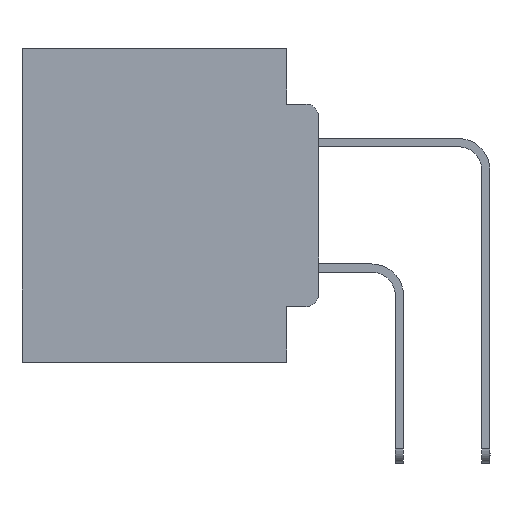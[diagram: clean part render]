
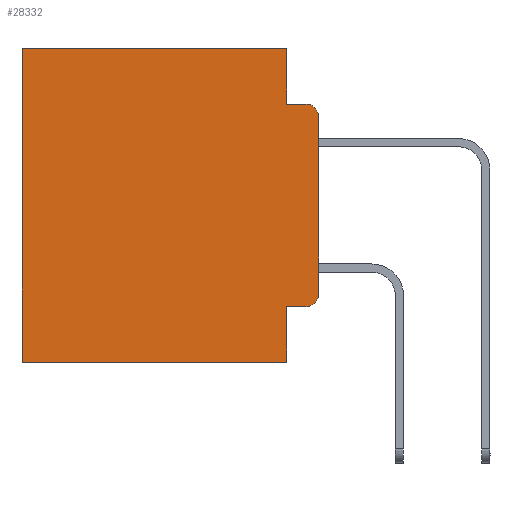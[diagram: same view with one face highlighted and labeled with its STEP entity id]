
A CAD part, left-side view. The second image highlights one B-rep face of the part: STEP entity #28332.
In plain terms, the highlighted planar face has unit normal (-1, 0, 0).
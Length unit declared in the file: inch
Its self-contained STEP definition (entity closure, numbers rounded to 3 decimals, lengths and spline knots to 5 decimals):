
#144 = LINE ( 'NONE', #2661, #5308 ) ;
#351 = VECTOR ( 'NONE', #19358, 39.37008 ) ;
#422 = LINE ( 'NONE', #11580, #24230 ) ;
#603 = EDGE_CURVE ( 'NONE', #9989, #10179, #6033, .T. ) ;
#659 = VERTEX_POINT ( 'NONE', #17639 ) ;
#731 = CARTESIAN_POINT ( 'NONE',  ( 0.298, 0.02, -0.3915 ) ) ;
#874 = VERTEX_POINT ( 'NONE', #2726 ) ;
#1506 = ORIENTED_EDGE ( 'NONE', *, *, #21153, .F. ) ;
#1819 = EDGE_LOOP ( 'NONE', ( #4537, #8935, #4600, #10059, #7791, #8073, #1506, #4955, #15226, #27487 ) ) ;
#2366 = DIRECTION ( 'NONE',  ( 0., 0., -1. ) ) ;
#2438 = DIRECTION ( 'NONE',  ( -1., 0., 0. ) ) ;
#2661 = CARTESIAN_POINT ( 'NONE',  ( 0.298, 0.051, 0. ) ) ;
#2663 = CARTESIAN_POINT ( 'NONE',  ( 0.298, 0., -0.1085 ) ) ;
#2726 = CARTESIAN_POINT ( 'NONE',  ( 0.298, 0.02, -0.4115 ) ) ;
#3197 = EDGE_CURVE ( 'NONE', #4149, #874, #23065, .T. ) ;
#3480 = CARTESIAN_POINT ( 'NONE',  ( 0.298, 0.473, 0. ) ) ;
#3643 = CARTESIAN_POINT ( 'NONE',  ( 0.298, 0.051, 0. ) ) ;
#4064 = VERTEX_POINT ( 'NONE', #20189 ) ;
#4145 = CARTESIAN_POINT ( 'NONE',  ( 0.298, 0., 0. ) ) ;
#4149 = VERTEX_POINT ( 'NONE', #6026 ) ;
#4158 = AXIS2_PLACEMENT_3D ( 'NONE', #731, #27908, #25831 ) ;
#4445 = CARTESIAN_POINT ( 'NONE',  ( 0.298, 0.473, 0. ) ) ;
#4537 = ORIENTED_EDGE ( 'NONE', *, *, #15327, .F. ) ;
#4600 = ORIENTED_EDGE ( 'NONE', *, *, #6429, .F. ) ;
#4626 = VERTEX_POINT ( 'NONE', #19662 ) ;
#4955 = ORIENTED_EDGE ( 'NONE', *, *, #25399, .F. ) ;
#5117 = CARTESIAN_POINT ( 'NONE',  ( 0.298, 0.02, -0.1085 ) ) ;
#5127 = EDGE_CURVE ( 'NONE', #9989, #21278, #16675, .T. ) ;
#5308 = VECTOR ( 'NONE', #2366, 39.37008 ) ;
#6026 = CARTESIAN_POINT ( 'NONE',  ( 0.298, 0.051, -0.4115 ) ) ;
#6033 = LINE ( 'NONE', #3643, #16654 ) ;
#6048 = CIRCLE ( 'NONE', #15077, 0.02 ) ;
#6429 = EDGE_CURVE ( 'NONE', #10179, #659, #422, .T. ) ;
#7589 = EDGE_CURVE ( 'NONE', #21278, #4064, #23687, .T. ) ;
#7630 = CARTESIAN_POINT ( 'NONE',  ( 0.298, 0., -0.5 ) ) ;
#7791 = ORIENTED_EDGE ( 'NONE', *, *, #5127, .T. ) ;
#8073 = ORIENTED_EDGE ( 'NONE', *, *, #7589, .T. ) ;
#8935 = ORIENTED_EDGE ( 'NONE', *, *, #19251, .T. ) ;
#9487 = DIRECTION ( 'NONE',  ( 0., -1., 0. ) ) ;
#9989 = VERTEX_POINT ( 'NONE', #18097 ) ;
#10059 = ORIENTED_EDGE ( 'NONE', *, *, #603, .F. ) ;
#10088 = VECTOR ( 'NONE', #12571, 39.37008 ) ;
#10179 = VERTEX_POINT ( 'NONE', #14681 ) ;
#10847 = CARTESIAN_POINT ( 'NONE',  ( 0.298, 0., 0. ) ) ;
#11580 = CARTESIAN_POINT ( 'NONE',  ( 0.298, 0.051, -0.0885 ) ) ;
#11797 = VERTEX_POINT ( 'NONE', #2663 ) ;
#12571 = DIRECTION ( 'NONE',  ( 0., 0., -1. ) ) ;
#14179 = CIRCLE ( 'NONE', #4158, 0.02 ) ;
#14202 = DIRECTION ( 'NONE',  ( 0., -1., 0. ) ) ;
#14396 = AXIS2_PLACEMENT_3D ( 'NONE', #4145, #21985, #19781 ) ;
#14681 = CARTESIAN_POINT ( 'NONE',  ( 0.298, 0.051, -0.0885 ) ) ;
#15010 = DIRECTION ( 'NONE',  ( 0., 0., -1. ) ) ;
#15077 = AXIS2_PLACEMENT_3D ( 'NONE', #5117, #2438, #27533 ) ;
#15092 = EDGE_CURVE ( 'NONE', #874, #27050, #14179, .T. ) ;
#15226 = ORIENTED_EDGE ( 'NONE', *, *, #3197, .T. ) ;
#15327 = EDGE_CURVE ( 'NONE', #11797, #27050, #17674, .T. ) ;
#16654 = VECTOR ( 'NONE', #27754, 39.37008 ) ;
#16675 = LINE ( 'NONE', #25716, #19917 ) ;
#17639 = CARTESIAN_POINT ( 'NONE',  ( 0.298, 0.02, -0.0885 ) ) ;
#17674 = LINE ( 'NONE', #10847, #18922 ) ;
#18097 = CARTESIAN_POINT ( 'NONE',  ( 0.298, 0.051, 0. ) ) ;
#18922 = VECTOR ( 'NONE', #15010, 39.37008 ) ;
#19079 = LINE ( 'NONE', #7630, #351 ) ;
#19251 = EDGE_CURVE ( 'NONE', #11797, #659, #6048, .T. ) ;
#19358 = DIRECTION ( 'NONE',  ( 0., 1., 0. ) ) ;
#19662 = CARTESIAN_POINT ( 'NONE',  ( 0.298, 0.051, -0.5 ) ) ;
#19781 = DIRECTION ( 'NONE',  ( 0., 0., -1. ) ) ;
#19917 = VECTOR ( 'NONE', #23477, 39.37008 ) ;
#20189 = CARTESIAN_POINT ( 'NONE',  ( 0.298, 0.473, -0.5 ) ) ;
#21153 = EDGE_CURVE ( 'NONE', #4626, #4064, #19079, .T. ) ;
#21278 = VERTEX_POINT ( 'NONE', #4445 ) ;
#21834 = CARTESIAN_POINT ( 'NONE',  ( 0.298, 0., -0.3915 ) ) ;
#21985 = DIRECTION ( 'NONE',  ( 1., 0., 0. ) ) ;
#23065 = LINE ( 'NONE', #27515, #27954 ) ;
#23477 = DIRECTION ( 'NONE',  ( 0., 1., 0. ) ) ;
#23687 = LINE ( 'NONE', #3480, #10088 ) ;
#24230 = VECTOR ( 'NONE', #9487, 39.37008 ) ;
#24627 = PLANE ( 'NONE',  #14396 ) ;
#24916 = FACE_OUTER_BOUND ( 'NONE', #1819, .T. ) ;
#25399 = EDGE_CURVE ( 'NONE', #4149, #4626, #144, .T. ) ;
#25716 = CARTESIAN_POINT ( 'NONE',  ( 0.298, 0., 0. ) ) ;
#25831 = DIRECTION ( 'NONE',  ( 0., 0., -1. ) ) ;
#27050 = VERTEX_POINT ( 'NONE', #21834 ) ;
#27487 = ORIENTED_EDGE ( 'NONE', *, *, #15092, .T. ) ;
#27515 = CARTESIAN_POINT ( 'NONE',  ( 0.298, 0.051, -0.4115 ) ) ;
#27533 = DIRECTION ( 'NONE',  ( 0., 0., -1. ) ) ;
#27754 = DIRECTION ( 'NONE',  ( 0., 0., -1. ) ) ;
#27908 = DIRECTION ( 'NONE',  ( -1., 0., 0. ) ) ;
#27954 = VECTOR ( 'NONE', #14202, 39.37008 ) ;
#28332 = ADVANCED_FACE ( 'NONE', ( #24916 ), #24627, .F. ) ;
